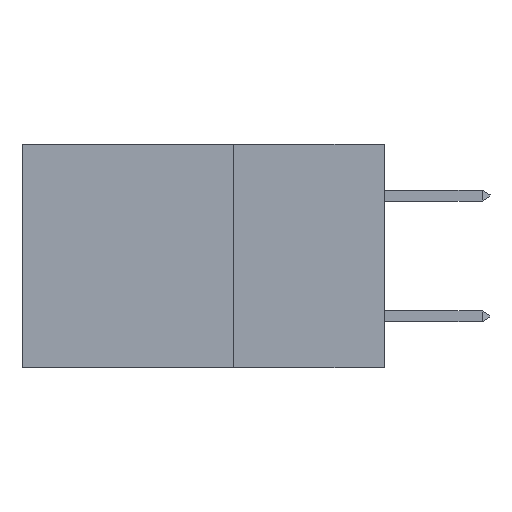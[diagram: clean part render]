
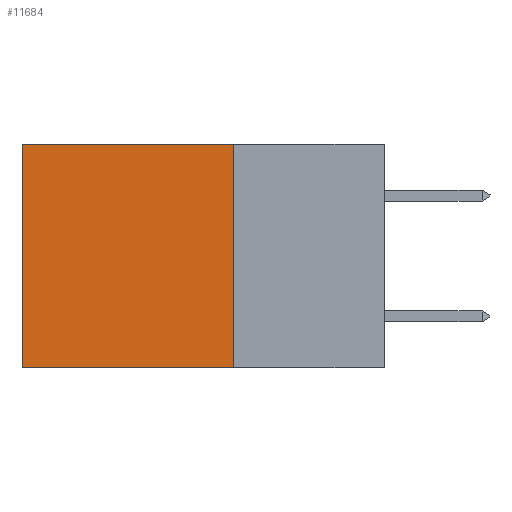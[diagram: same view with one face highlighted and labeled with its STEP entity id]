
A CAD part, left-side view. The second image highlights one B-rep face of the part: STEP entity #11684.
In plain terms, the highlighted planar face has unit normal (-1, 0, 0).
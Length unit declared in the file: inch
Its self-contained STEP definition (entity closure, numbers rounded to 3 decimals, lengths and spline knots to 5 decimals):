
#106 = VERTEX_POINT ( 'NONE', #3319 ) ;
#1154 = VECTOR ( 'NONE', #34017, 39.37008 ) ;
#3319 = CARTESIAN_POINT ( 'NONE',  ( 0.2875, 0.6, 0. ) ) ;
#3911 = LINE ( 'NONE', #29228, #33353 ) ;
#5737 = CARTESIAN_POINT ( 'NONE',  ( 0.2875, 0.25, 0. ) ) ;
#7391 = EDGE_CURVE ( 'NONE', #106, #14609, #32555, .T. ) ;
#8708 = DIRECTION ( 'NONE',  ( 0., 0., -1. ) ) ;
#10161 = ORIENTED_EDGE ( 'NONE', *, *, #14017, .T. ) ;
#11107 = CARTESIAN_POINT ( 'NONE',  ( 0.2875, 0.25, 0. ) ) ;
#11684 = ADVANCED_FACE ( 'NONE', ( #23457 ), #25160, .F. ) ;
#13054 = CARTESIAN_POINT ( 'NONE',  ( 0.2875, 0.25, -0.37 ) ) ;
#13720 = VERTEX_POINT ( 'NONE', #19532 ) ;
#14017 = EDGE_CURVE ( 'NONE', #35998, #106, #3911, .T. ) ;
#14609 = VERTEX_POINT ( 'NONE', #20345 ) ;
#16332 = AXIS2_PLACEMENT_3D ( 'NONE', #33592, #16712, #36371 ) ;
#16712 = DIRECTION ( 'NONE',  ( 1., 0., 0. ) ) ;
#17836 = DIRECTION ( 'NONE',  ( 0., 1., 0. ) ) ;
#18506 = ORIENTED_EDGE ( 'NONE', *, *, #7391, .T. ) ;
#19532 = CARTESIAN_POINT ( 'NONE',  ( 0.2875, 0.25, -0.37 ) ) ;
#20345 = CARTESIAN_POINT ( 'NONE',  ( 0.2875, 0.6, -0.37 ) ) ;
#23457 = FACE_OUTER_BOUND ( 'NONE', #32520, .T. ) ;
#24694 = ORIENTED_EDGE ( 'NONE', *, *, #33794, .F. ) ;
#25160 = PLANE ( 'NONE',  #16332 ) ;
#26987 = VECTOR ( 'NONE', #30096, 39.37008 ) ;
#27875 = LINE ( 'NONE', #13054, #26987 ) ;
#29228 = CARTESIAN_POINT ( 'NONE',  ( 0.2875, 0.25, 0. ) ) ;
#30096 = DIRECTION ( 'NONE',  ( 0., 1., 0. ) ) ;
#30718 = VECTOR ( 'NONE', #8708, 39.37008 ) ;
#31241 = CARTESIAN_POINT ( 'NONE',  ( 0.2875, 0.6, 0. ) ) ;
#31583 = LINE ( 'NONE', #5737, #30718 ) ;
#32520 = EDGE_LOOP ( 'NONE', ( #18506, #34359, #24694, #10161 ) ) ;
#32555 = LINE ( 'NONE', #31241, #1154 ) ;
#33353 = VECTOR ( 'NONE', #17836, 39.37008 ) ;
#33592 = CARTESIAN_POINT ( 'NONE',  ( 0.2875, 0.25, 0. ) ) ;
#33794 = EDGE_CURVE ( 'NONE', #35998, #13720, #31583, .T. ) ;
#34017 = DIRECTION ( 'NONE',  ( 0., 0., -1. ) ) ;
#34359 = ORIENTED_EDGE ( 'NONE', *, *, #36447, .F. ) ;
#35998 = VERTEX_POINT ( 'NONE', #11107 ) ;
#36371 = DIRECTION ( 'NONE',  ( 0., 0., -1. ) ) ;
#36447 = EDGE_CURVE ( 'NONE', #13720, #14609, #27875, .T. ) ;
